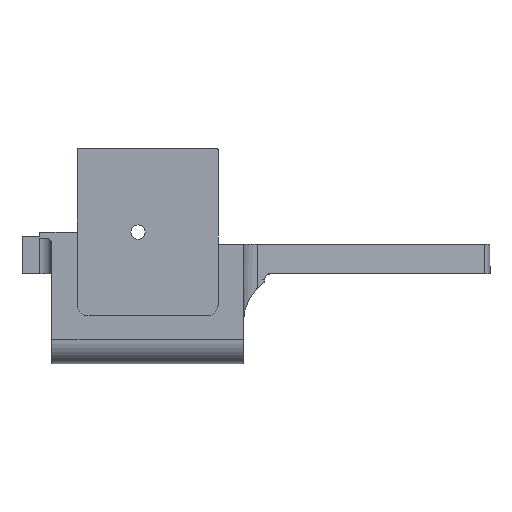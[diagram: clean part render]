
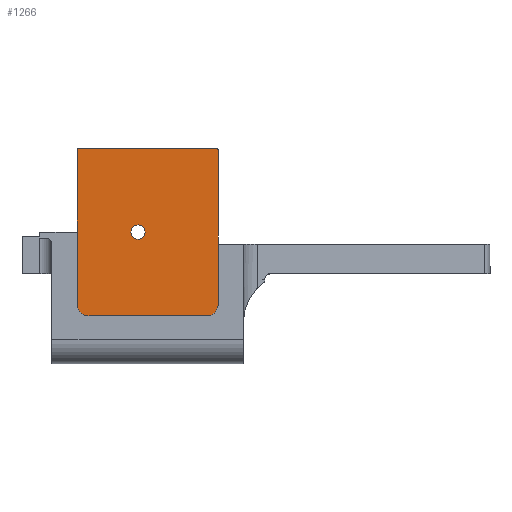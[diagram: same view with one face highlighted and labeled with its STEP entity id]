
A CAD part, left-side view. The second image highlights one B-rep face of the part: STEP entity #1266.
In plain terms, the highlighted planar face has unit normal (-1, 0, 0).
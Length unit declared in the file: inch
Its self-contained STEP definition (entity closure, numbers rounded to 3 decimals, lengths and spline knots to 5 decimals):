
#46 = CARTESIAN_POINT ( 'NONE',  ( 0.7, 1.39, 0.4 ) ) ;
#58 = CARTESIAN_POINT ( 'NONE',  ( 0.7, 1.39, 1.78 ) ) ;
#110 = VERTEX_POINT ( 'NONE', #4170 ) ;
#176 = LINE ( 'NONE', #3598, #1291 ) ;
#249 = VERTEX_POINT ( 'NONE', #1339 ) ;
#315 = LINE ( 'NONE', #1662, #6341 ) ;
#414 = DIRECTION ( 'NONE',  ( -1., 0., 0. ) ) ;
#460 = ORIENTED_EDGE ( 'NONE', *, *, #4143, .T. ) ;
#614 = LINE ( 'NONE', #5436, #1198 ) ;
#704 = VECTOR ( 'NONE', #1472, 39.37008 ) ;
#758 = ORIENTED_EDGE ( 'NONE', *, *, #5522, .T. ) ;
#815 = VERTEX_POINT ( 'NONE', #6271 ) ;
#841 = ORIENTED_EDGE ( 'NONE', *, *, #4510, .T. ) ;
#881 = CARTESIAN_POINT ( 'NONE',  ( 0.7, 0.23, 1.78 ) ) ;
#1096 = EDGE_CURVE ( 'NONE', #5822, #6073, #4557, .T. ) ;
#1198 = VECTOR ( 'NONE', #1935, 39.37008 ) ;
#1266 = ADVANCED_FACE ( 'NONE', ( #3128, #3628 ), #4359, .T. ) ;
#1291 = VECTOR ( 'NONE', #4610, 39.37008 ) ;
#1337 = DIRECTION ( 'NONE',  ( 0., 0., -1. ) ) ;
#1339 = CARTESIAN_POINT ( 'NONE',  ( 0.7, 0.6, 0.4 ) ) ;
#1373 = DIRECTION ( 'NONE',  ( -1., 0., 0. ) ) ;
#1392 = AXIS2_PLACEMENT_3D ( 'NONE', #3405, #1373, #3927 ) ;
#1472 = DIRECTION ( 'NONE',  ( 0., 0., -1. ) ) ;
#1501 = EDGE_CURVE ( 'NONE', #815, #3884, #315, .T. ) ;
#1514 = ORIENTED_EDGE ( 'NONE', *, *, #2302, .T. ) ;
#1599 = ORIENTED_EDGE ( 'NONE', *, *, #1991, .F. ) ;
#1621 = EDGE_CURVE ( 'NONE', #1850, #5679, #3537, .T. ) ;
#1662 = CARTESIAN_POINT ( 'NONE',  ( 0.7, 0.21, 1.78 ) ) ;
#1681 = ORIENTED_EDGE ( 'NONE', *, *, #1096, .T. ) ;
#1721 = DIRECTION ( 'NONE',  ( 0., 0., 1. ) ) ;
#1773 = VERTEX_POINT ( 'NONE', #6010 ) ;
#1794 = CARTESIAN_POINT ( 'NONE',  ( 0.7, 1.37, 1.8 ) ) ;
#1836 = CARTESIAN_POINT ( 'NONE',  ( 0.7, 0.88094, 1.04094 ) ) ;
#1850 = VERTEX_POINT ( 'NONE', #3065 ) ;
#1894 = DIRECTION ( 'NONE',  ( -1., 0., 0. ) ) ;
#1935 = DIRECTION ( 'NONE',  ( 0., 0., -1. ) ) ;
#1969 = EDGE_LOOP ( 'NONE', ( #3362, #3079, #5022, #841, #1514, #1681, #3857, #460, #2438, #2628, #758, #2447, #5786, #2900 ) ) ;
#1991 = EDGE_CURVE ( 'NONE', #5679, #1850, #5932, .T. ) ;
#2094 = CARTESIAN_POINT ( 'NONE',  ( 0.7, 1.37, 1.78 ) ) ;
#2100 = CIRCLE ( 'NONE', #5626, 0.02 ) ;
#2101 = CARTESIAN_POINT ( 'NONE',  ( 0.7, 1.29, 0.4 ) ) ;
#2149 = DIRECTION ( 'NONE',  ( -1., 0., 0. ) ) ;
#2219 = VERTEX_POINT ( 'NONE', #4844 ) ;
#2242 = DIRECTION ( 'NONE',  ( 0., 0., 1. ) ) ;
#2264 = DIRECTION ( 'NONE',  ( -1., 0., 0. ) ) ;
#2302 = EDGE_CURVE ( 'NONE', #5129, #5822, #2100, .T. ) ;
#2355 = LINE ( 'NONE', #4972, #3776 ) ;
#2367 = LINE ( 'NONE', #5397, #704 ) ;
#2392 = LINE ( 'NONE', #46, #4198 ) ;
#2393 = DIRECTION ( 'NONE',  ( 0., 0., 1. ) ) ;
#2405 = CARTESIAN_POINT ( 'NONE',  ( 0.7, 0., 0.2 ) ) ;
#2438 = ORIENTED_EDGE ( 'NONE', *, *, #4069, .T. ) ;
#2447 = ORIENTED_EDGE ( 'NONE', *, *, #6297, .T. ) ;
#2499 = EDGE_CURVE ( 'NONE', #2219, #110, #4543, .T. ) ;
#2532 = CARTESIAN_POINT ( 'NONE',  ( 0.7, 1.37, 1.8 ) ) ;
#2628 = ORIENTED_EDGE ( 'NONE', *, *, #5983, .T. ) ;
#2629 = AXIS2_PLACEMENT_3D ( 'NONE', #2791, #414, #4412 ) ;
#2695 = AXIS2_PLACEMENT_3D ( 'NONE', #3383, #1894, #2393 ) ;
#2755 = CARTESIAN_POINT ( 'NONE',  ( 0.7, 1.39, 0.4 ) ) ;
#2791 = CARTESIAN_POINT ( 'NONE',  ( 0.7, 0.88094, 1.1 ) ) ;
#2823 = CIRCLE ( 'NONE', #2695, 0.1 ) ;
#2900 = ORIENTED_EDGE ( 'NONE', *, *, #3297, .F. ) ;
#3065 = CARTESIAN_POINT ( 'NONE',  ( 0.7, 0.88094, 1.15906 ) ) ;
#3079 = ORIENTED_EDGE ( 'NONE', *, *, #4821, .T. ) ;
#3097 = VECTOR ( 'NONE', #3742, 39.37008 ) ;
#3128 = FACE_OUTER_BOUND ( 'NONE', #1969, .T. ) ;
#3159 = VERTEX_POINT ( 'NONE', #5205 ) ;
#3174 = DIRECTION ( 'NONE',  ( 0., 0., 1. ) ) ;
#3233 = DIRECTION ( 'NONE',  ( -1., 0., 0. ) ) ;
#3297 = EDGE_CURVE ( 'NONE', #249, #2219, #2367, .T. ) ;
#3320 = DIRECTION ( 'NONE',  ( 0., 0., 1. ) ) ;
#3362 = ORIENTED_EDGE ( 'NONE', *, *, #3563, .T. ) ;
#3383 = CARTESIAN_POINT ( 'NONE',  ( 0.7, 1.29, 0.5 ) ) ;
#3405 = CARTESIAN_POINT ( 'NONE',  ( 0.7, 0., 0.4 ) ) ;
#3537 = CIRCLE ( 'NONE', #2629, 0.05906 ) ;
#3553 = EDGE_CURVE ( 'NONE', #6073, #5178, #6270, .T. ) ;
#3563 = EDGE_CURVE ( 'NONE', #249, #5281, #176, .T. ) ;
#3598 = CARTESIAN_POINT ( 'NONE',  ( 0.7, 0.21, 0.4 ) ) ;
#3601 = CARTESIAN_POINT ( 'NONE',  ( 0.7, 0.21, 1.78 ) ) ;
#3628 = FACE_BOUND ( 'NONE', #6198, .T. ) ;
#3642 = ORIENTED_EDGE ( 'NONE', *, *, #1621, .F. ) ;
#3742 = DIRECTION ( 'NONE',  ( 0., 0., -1. ) ) ;
#3769 = CARTESIAN_POINT ( 'NONE',  ( 0.7, 0.31, 0.5 ) ) ;
#3776 = VECTOR ( 'NONE', #4477, 39.37008 ) ;
#3804 = AXIS2_PLACEMENT_3D ( 'NONE', #3769, #2264, #2242 ) ;
#3847 = VECTOR ( 'NONE', #6360, 39.37008 ) ;
#3857 = ORIENTED_EDGE ( 'NONE', *, *, #3553, .T. ) ;
#3884 = VERTEX_POINT ( 'NONE', #5059 ) ;
#3927 = DIRECTION ( 'NONE',  ( 0., 0., 1. ) ) ;
#4069 = EDGE_CURVE ( 'NONE', #1773, #6106, #5781, .T. ) ;
#4123 = AXIS2_PLACEMENT_3D ( 'NONE', #2094, #2149, #4674 ) ;
#4143 = EDGE_CURVE ( 'NONE', #5178, #1773, #2392, .T. ) ;
#4170 = CARTESIAN_POINT ( 'NONE',  ( 0.7, 1., 0.2 ) ) ;
#4198 = VECTOR ( 'NONE', #5982, 39.37008 ) ;
#4295 = DIRECTION ( 'NONE',  ( -1., 0., 0. ) ) ;
#4359 = PLANE ( 'NONE',  #1392 ) ;
#4412 = DIRECTION ( 'NONE',  ( 0., 0., 1. ) ) ;
#4477 = DIRECTION ( 'NONE',  ( 0., -1., 0. ) ) ;
#4510 = EDGE_CURVE ( 'NONE', #3884, #5129, #5773, .T. ) ;
#4543 = LINE ( 'NONE', #2405, #3847 ) ;
#4557 = LINE ( 'NONE', #1794, #6043 ) ;
#4610 = DIRECTION ( 'NONE',  ( 0., -1., 0. ) ) ;
#4674 = DIRECTION ( 'NONE',  ( 0., 0., -1. ) ) ;
#4821 = EDGE_CURVE ( 'NONE', #5281, #815, #5974, .T. ) ;
#4844 = CARTESIAN_POINT ( 'NONE',  ( 0.7, 0.6, 0.2 ) ) ;
#4914 = VECTOR ( 'NONE', #1721, 39.37008 ) ;
#4972 = CARTESIAN_POINT ( 'NONE',  ( 0.7, 0.21, 0.4 ) ) ;
#5011 = CARTESIAN_POINT ( 'NONE',  ( 0.7, 0.23, 1.8 ) ) ;
#5022 = ORIENTED_EDGE ( 'NONE', *, *, #1501, .T. ) ;
#5059 = CARTESIAN_POINT ( 'NONE',  ( 0.7, 0.21, 1. ) ) ;
#5107 = CARTESIAN_POINT ( 'NONE',  ( 0.7, 0.31, 0.4 ) ) ;
#5129 = VERTEX_POINT ( 'NONE', #3601 ) ;
#5171 = CARTESIAN_POINT ( 'NONE',  ( 0.7, 0.21, 1.78 ) ) ;
#5178 = VERTEX_POINT ( 'NONE', #58 ) ;
#5205 = CARTESIAN_POINT ( 'NONE',  ( 0.7, 1., 0.4 ) ) ;
#5281 = VERTEX_POINT ( 'NONE', #5107 ) ;
#5287 = VERTEX_POINT ( 'NONE', #2101 ) ;
#5397 = CARTESIAN_POINT ( 'NONE',  ( 0.7, 0.6, 0.4 ) ) ;
#5436 = CARTESIAN_POINT ( 'NONE',  ( 0.7, 1., 0.4 ) ) ;
#5522 = EDGE_CURVE ( 'NONE', #5287, #3159, #2355, .T. ) ;
#5626 = AXIS2_PLACEMENT_3D ( 'NONE', #881, #4295, #1337 ) ;
#5679 = VERTEX_POINT ( 'NONE', #1836 ) ;
#5773 = LINE ( 'NONE', #5171, #4914 ) ;
#5781 = LINE ( 'NONE', #2755, #3097 ) ;
#5786 = ORIENTED_EDGE ( 'NONE', *, *, #2499, .F. ) ;
#5822 = VERTEX_POINT ( 'NONE', #5011 ) ;
#5834 = CARTESIAN_POINT ( 'NONE',  ( 0.7, 0.88094, 1.1 ) ) ;
#5932 = CIRCLE ( 'NONE', #6306, 0.05906 ) ;
#5974 = CIRCLE ( 'NONE', #3804, 0.1 ) ;
#5982 = DIRECTION ( 'NONE',  ( 0., 0., -1. ) ) ;
#5983 = EDGE_CURVE ( 'NONE', #6106, #5287, #2823, .T. ) ;
#6010 = CARTESIAN_POINT ( 'NONE',  ( 0.7, 1.39, 1.1 ) ) ;
#6035 = CARTESIAN_POINT ( 'NONE',  ( 0.7, 1.39, 0.5 ) ) ;
#6043 = VECTOR ( 'NONE', #6215, 39.37008 ) ;
#6073 = VERTEX_POINT ( 'NONE', #2532 ) ;
#6106 = VERTEX_POINT ( 'NONE', #6035 ) ;
#6198 = EDGE_LOOP ( 'NONE', ( #3642, #1599 ) ) ;
#6215 = DIRECTION ( 'NONE',  ( 0., 1., 0. ) ) ;
#6270 = CIRCLE ( 'NONE', #4123, 0.02 ) ;
#6271 = CARTESIAN_POINT ( 'NONE',  ( 0.7, 0.21, 0.5 ) ) ;
#6297 = EDGE_CURVE ( 'NONE', #3159, #110, #614, .T. ) ;
#6306 = AXIS2_PLACEMENT_3D ( 'NONE', #5834, #3233, #3320 ) ;
#6341 = VECTOR ( 'NONE', #3174, 39.37008 ) ;
#6360 = DIRECTION ( 'NONE',  ( 0., 1., 0. ) ) ;
